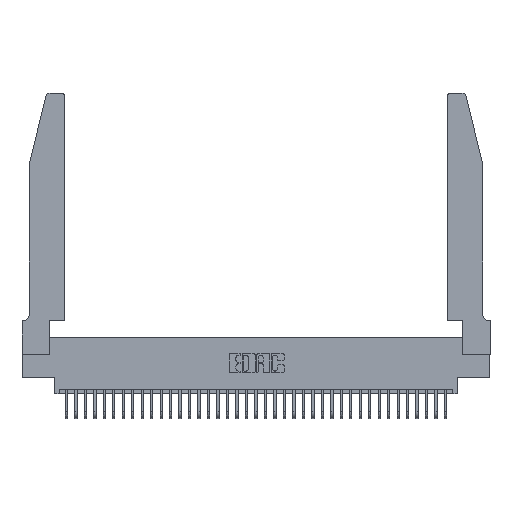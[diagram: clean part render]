
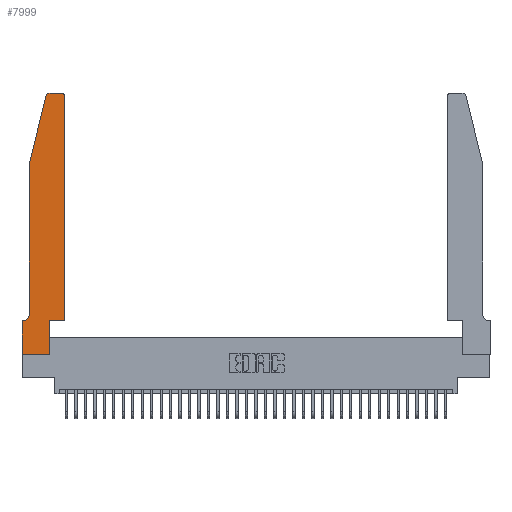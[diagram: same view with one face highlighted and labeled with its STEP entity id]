
A CAD part, top view. The second image highlights one B-rep face of the part: STEP entity #7999.
In plain terms, the highlighted planar face has unit normal (0, 0, 1).
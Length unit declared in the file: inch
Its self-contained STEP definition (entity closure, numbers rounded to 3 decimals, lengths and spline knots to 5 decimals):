
#296 = VERTEX_POINT ( 'NONE', #27542 ) ;
#1336 = ORIENTED_EDGE ( 'NONE', *, *, #11765, .T. ) ;
#1552 = EDGE_CURVE ( 'NONE', #27569, #296, #27091, .T. ) ;
#1793 = DIRECTION ( 'NONE',  ( -1., 0., 0. ) ) ;
#1994 = LINE ( 'NONE', #12692, #27126 ) ;
#2917 = VECTOR ( 'NONE', #15780, 39.37008 ) ;
#2942 = DIRECTION ( 'NONE',  ( 1., 0., 0. ) ) ;
#3487 = DIRECTION ( 'NONE',  ( -1., 0., 0. ) ) ;
#3593 = VECTOR ( 'NONE', #37556, 39.37008 ) ;
#3604 = CIRCLE ( 'NONE', #29401, 0.03 ) ;
#4567 = LINE ( 'NONE', #13717, #3593 ) ;
#5302 = VERTEX_POINT ( 'NONE', #12035 ) ;
#5492 = VERTEX_POINT ( 'NONE', #18714 ) ;
#5620 = CARTESIAN_POINT ( 'NONE',  ( 0.4205, 2.72, 0.37 ) ) ;
#5888 = CARTESIAN_POINT ( 'NONE',  ( 0., 0.35, 0.37 ) ) ;
#6155 = CARTESIAN_POINT ( 'NONE',  ( 0.4505, 0.35, 0.37 ) ) ;
#6173 = CARTESIAN_POINT ( 'NONE',  ( 0., 0., 0.37 ) ) ;
#6939 = VECTOR ( 'NONE', #27340, 39.37008 ) ;
#7167 = CARTESIAN_POINT ( 'NONE',  ( 0.0055, 0.35, 0.37 ) ) ;
#7298 = DIRECTION ( 'NONE',  ( 0., 0., 1. ) ) ;
#7611 = VERTEX_POINT ( 'NONE', #13500 ) ;
#7999 = ADVANCED_FACE ( 'NONE', ( #8215 ), #18165, .T. ) ;
#8215 = FACE_OUTER_BOUND ( 'NONE', #16282, .T. ) ;
#8686 = DIRECTION ( 'NONE',  ( 1., 0., 0. ) ) ;
#9462 = LINE ( 'NONE', #20374, #25573 ) ;
#10316 = VERTEX_POINT ( 'NONE', #13998 ) ;
#10828 = CARTESIAN_POINT ( 'NONE',  ( 0.4505, 0.35, 0.37 ) ) ;
#11468 = EDGE_CURVE ( 'NONE', #7611, #5492, #23581, .T. ) ;
#11522 = EDGE_CURVE ( 'NONE', #10316, #31108, #14590, .T. ) ;
#11613 = CIRCLE ( 'NONE', #21747, 0.03 ) ;
#11765 = EDGE_CURVE ( 'NONE', #23211, #13032, #21216, .T. ) ;
#11847 = ORIENTED_EDGE ( 'NONE', *, *, #11522, .T. ) ;
#12035 = CARTESIAN_POINT ( 'NONE',  ( 0.4505, 2.72, 0.37 ) ) ;
#12354 = ORIENTED_EDGE ( 'NONE', *, *, #37323, .T. ) ;
#12523 = CARTESIAN_POINT ( 'NONE',  ( 0.0755, 0.35, 0.37 ) ) ;
#12692 = CARTESIAN_POINT ( 'NONE',  ( 0.0755, 2., 0.37 ) ) ;
#13032 = VERTEX_POINT ( 'NONE', #37968 ) ;
#13436 = ORIENTED_EDGE ( 'NONE', *, *, #1552, .T. ) ;
#13500 = CARTESIAN_POINT ( 'NONE',  ( 0.4205, 2.75, 0.37 ) ) ;
#13717 = CARTESIAN_POINT ( 'NONE',  ( 0.4505, 0.35, 0.37 ) ) ;
#13998 = CARTESIAN_POINT ( 'NONE',  ( 0.25487, 2.72718, 0.37 ) ) ;
#14590 = LINE ( 'NONE', #20169, #37406 ) ;
#15556 = VECTOR ( 'NONE', #1793, 39.37008 ) ;
#15780 = DIRECTION ( 'NONE',  ( 0., 1., 0. ) ) ;
#16282 = EDGE_LOOP ( 'NONE', ( #18049, #32424, #11847, #38219, #29136, #16462, #1336, #12354, #13436, #19774, #38742, #19601 ) ) ;
#16462 = ORIENTED_EDGE ( 'NONE', *, *, #18781, .T. ) ;
#17845 = CARTESIAN_POINT ( 'NONE',  ( 0.0055, 0.42, 0.37 ) ) ;
#18049 = ORIENTED_EDGE ( 'NONE', *, *, #11468, .T. ) ;
#18165 = PLANE ( 'NONE',  #33850 ) ;
#18714 = CARTESIAN_POINT ( 'NONE',  ( 0.284, 2.75, 0.37 ) ) ;
#18781 = EDGE_CURVE ( 'NONE', #29931, #23211, #19162, .T. ) ;
#19162 = LINE ( 'NONE', #12523, #34064 ) ;
#19601 = ORIENTED_EDGE ( 'NONE', *, *, #23335, .T. ) ;
#19774 = ORIENTED_EDGE ( 'NONE', *, *, #31225, .T. ) ;
#20042 = CARTESIAN_POINT ( 'NONE',  ( 0.2605, 2.75, 0.37 ) ) ;
#20169 = CARTESIAN_POINT ( 'NONE',  ( 0.0755, 2., 0.37 ) ) ;
#20374 = CARTESIAN_POINT ( 'NONE',  ( 0., 0., 0.37 ) ) ;
#20867 = DIRECTION ( 'NONE',  ( -1., 0., 0. ) ) ;
#21173 = DIRECTION ( 'NONE',  ( 0., 0., 1. ) ) ;
#21216 = LINE ( 'NONE', #6173, #6939 ) ;
#21330 = DIRECTION ( 'NONE',  ( 0., 1., 0. ) ) ;
#21747 = AXIS2_PLACEMENT_3D ( 'NONE', #5620, #26788, #8686 ) ;
#22052 = LINE ( 'NONE', #6155, #35938 ) ;
#22401 = EDGE_CURVE ( 'NONE', #5492, #10316, #3604, .T. ) ;
#23130 = VERTEX_POINT ( 'NONE', #28741 ) ;
#23211 = VERTEX_POINT ( 'NONE', #31994 ) ;
#23335 = EDGE_CURVE ( 'NONE', #5302, #7611, #11613, .T. ) ;
#23413 = DIRECTION ( 'NONE',  ( 1., 0., 0. ) ) ;
#23581 = LINE ( 'NONE', #20042, #15556 ) ;
#24370 = EDGE_CURVE ( 'NONE', #31108, #23130, #1994, .T. ) ;
#24890 = AXIS2_PLACEMENT_3D ( 'NONE', #17845, #38540, #20867 ) ;
#25428 = CARTESIAN_POINT ( 'NONE',  ( 0.284, 2.72, 0.37 ) ) ;
#25573 = VECTOR ( 'NONE', #23413, 39.37008 ) ;
#26353 = VERTEX_POINT ( 'NONE', #10828 ) ;
#26788 = DIRECTION ( 'NONE',  ( 0., 0., 1. ) ) ;
#27091 = LINE ( 'NONE', #36594, #2917 ) ;
#27126 = VECTOR ( 'NONE', #27734, 39.37008 ) ;
#27340 = DIRECTION ( 'NONE',  ( 0., -1., 0. ) ) ;
#27542 = CARTESIAN_POINT ( 'NONE',  ( 0.2865, 0.35, 0.37 ) ) ;
#27569 = VERTEX_POINT ( 'NONE', #37629 ) ;
#27734 = DIRECTION ( 'NONE',  ( 0., -1., 0. ) ) ;
#28432 = DIRECTION ( 'NONE',  ( 1., 0., 0. ) ) ;
#28741 = CARTESIAN_POINT ( 'NONE',  ( 0.0755, 0.42, 0.37 ) ) ;
#29136 = ORIENTED_EDGE ( 'NONE', *, *, #36117, .T. ) ;
#29401 = AXIS2_PLACEMENT_3D ( 'NONE', #25428, #7298, #28432 ) ;
#29931 = VERTEX_POINT ( 'NONE', #7167 ) ;
#31108 = VERTEX_POINT ( 'NONE', #34159 ) ;
#31225 = EDGE_CURVE ( 'NONE', #296, #26353, #4567, .T. ) ;
#31994 = CARTESIAN_POINT ( 'NONE',  ( 0., 0.35, 0.37 ) ) ;
#32424 = ORIENTED_EDGE ( 'NONE', *, *, #22401, .T. ) ;
#33850 = AXIS2_PLACEMENT_3D ( 'NONE', #5888, #21173, #2942 ) ;
#34064 = VECTOR ( 'NONE', #3487, 39.37008 ) ;
#34159 = CARTESIAN_POINT ( 'NONE',  ( 0.0755, 2., 0.37 ) ) ;
#34795 = EDGE_CURVE ( 'NONE', #26353, #5302, #22052, .T. ) ;
#34907 = CIRCLE ( 'NONE', #24890, 0.07 ) ;
#35938 = VECTOR ( 'NONE', #21330, 39.37008 ) ;
#36117 = EDGE_CURVE ( 'NONE', #23130, #29931, #34907, .T. ) ;
#36594 = CARTESIAN_POINT ( 'NONE',  ( 0.2865, 0.35, 0.37 ) ) ;
#37323 = EDGE_CURVE ( 'NONE', #13032, #27569, #9462, .T. ) ;
#37406 = VECTOR ( 'NONE', #37860, 39.37008 ) ;
#37556 = DIRECTION ( 'NONE',  ( 1., 0., 0. ) ) ;
#37629 = CARTESIAN_POINT ( 'NONE',  ( 0.2865, 0., 0.37 ) ) ;
#37860 = DIRECTION ( 'NONE',  ( -0.239, -0.971, 0. ) ) ;
#37968 = CARTESIAN_POINT ( 'NONE',  ( 0., 0., 0.37 ) ) ;
#38219 = ORIENTED_EDGE ( 'NONE', *, *, #24370, .T. ) ;
#38540 = DIRECTION ( 'NONE',  ( 0., 0., -1. ) ) ;
#38742 = ORIENTED_EDGE ( 'NONE', *, *, #34795, .T. ) ;
